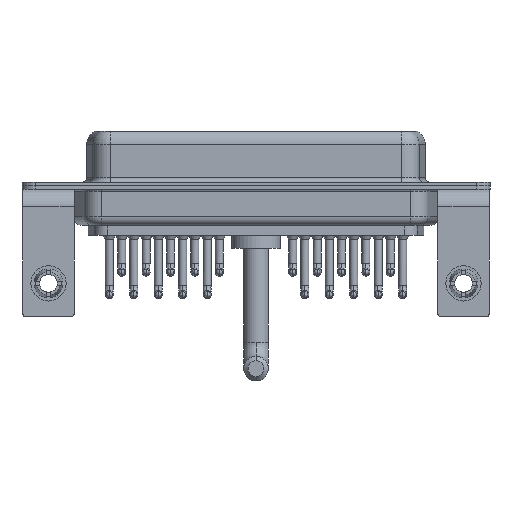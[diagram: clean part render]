
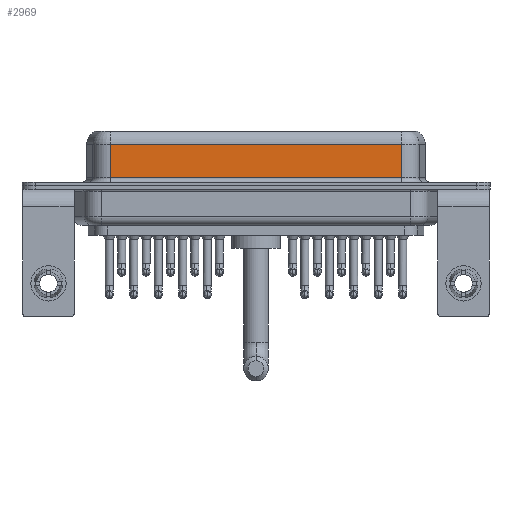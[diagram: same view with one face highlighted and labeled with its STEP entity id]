
A CAD part, front view. The second image highlights one B-rep face of the part: STEP entity #2969.
In plain terms, the highlighted planar face has unit normal (0, -1, 0).
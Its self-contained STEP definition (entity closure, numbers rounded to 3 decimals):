
#172 = VERTEX_POINT ( 'NONE', #20106 ) ;
#276 = VERTEX_POINT ( 'NONE', #13157 ) ;
#303 = LINE ( 'NONE', #17796, #21125 ) ;
#767 = DIRECTION ( 'NONE',  ( 1., 0., 0. ) ) ;
#903 = CARTESIAN_POINT ( 'NONE',  ( 40.037, -3.95, 0.9 ) ) ;
#1067 = EDGE_CURVE ( 'NONE', #1983, #21295, #8506, .T. ) ;
#1983 = VERTEX_POINT ( 'NONE', #6900 ) ;
#2906 = DIRECTION ( 'NONE',  ( 0., 0., 1. ) ) ;
#2969 = ADVANCED_FACE ( 'NONE', ( #8483 ), #8863, .F. ) ;
#3280 = DIRECTION ( 'NONE',  ( 0., 0., -1. ) ) ;
#3337 = ORIENTED_EDGE ( 'NONE', *, *, #1067, .T. ) ;
#3931 = DIRECTION ( 'NONE',  ( 0., 0., -1. ) ) ;
#4590 = ORIENTED_EDGE ( 'NONE', *, *, #18369, .T. ) ;
#5949 = CARTESIAN_POINT ( 'NONE',  ( 40.037, -3.95, 6.4 ) ) ;
#6900 = CARTESIAN_POINT ( 'NONE',  ( 7.013, -3.95, 0.9 ) ) ;
#6954 = ORIENTED_EDGE ( 'NONE', *, *, #9127, .F. ) ;
#7462 = LINE ( 'NONE', #24430, #7923 ) ;
#7923 = VECTOR ( 'NONE', #3280, 1000. ) ;
#8483 = FACE_OUTER_BOUND ( 'NONE', #24000, .T. ) ;
#8506 = LINE ( 'NONE', #903, #12072 ) ;
#8863 = PLANE ( 'NONE',  #10877 ) ;
#9127 = EDGE_CURVE ( 'NONE', #172, #21295, #13431, .T. ) ;
#10877 = AXIS2_PLACEMENT_3D ( 'NONE', #18227, #16576, #2906 ) ;
#12072 = VECTOR ( 'NONE', #767, 1000. ) ;
#13157 = CARTESIAN_POINT ( 'NONE',  ( 7.013, -3.95, 4.65 ) ) ;
#13431 = LINE ( 'NONE', #5949, #19116 ) ;
#16576 = DIRECTION ( 'NONE',  ( 0., 1., 0. ) ) ;
#17641 = ORIENTED_EDGE ( 'NONE', *, *, #18894, .T. ) ;
#17796 = CARTESIAN_POINT ( 'NONE',  ( 40.037, -3.95, 4.65 ) ) ;
#18227 = CARTESIAN_POINT ( 'NONE',  ( 40.037, -3.95, 6.4 ) ) ;
#18369 = EDGE_CURVE ( 'NONE', #276, #1983, #7462, .T. ) ;
#18894 = EDGE_CURVE ( 'NONE', #172, #276, #303, .T. ) ;
#19116 = VECTOR ( 'NONE', #3931, 1000. ) ;
#20106 = CARTESIAN_POINT ( 'NONE',  ( 40.037, -3.95, 4.65 ) ) ;
#21125 = VECTOR ( 'NONE', #21229, 1000. ) ;
#21229 = DIRECTION ( 'NONE',  ( -1., 0., 0. ) ) ;
#21295 = VERTEX_POINT ( 'NONE', #24517 ) ;
#24000 = EDGE_LOOP ( 'NONE', ( #6954, #17641, #4590, #3337 ) ) ;
#24430 = CARTESIAN_POINT ( 'NONE',  ( 7.013, -3.95, 6.4 ) ) ;
#24517 = CARTESIAN_POINT ( 'NONE',  ( 40.037, -3.95, 0.9 ) ) ;
